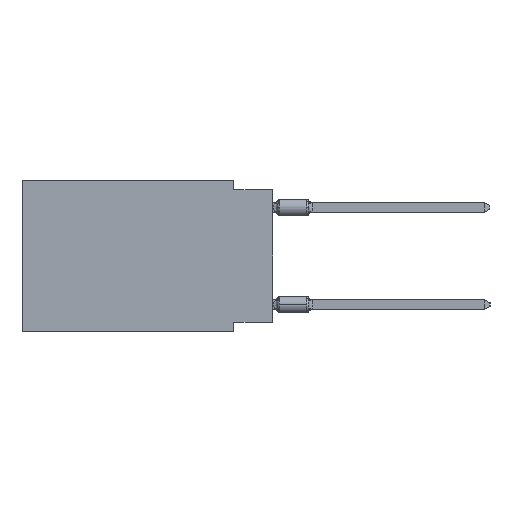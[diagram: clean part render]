
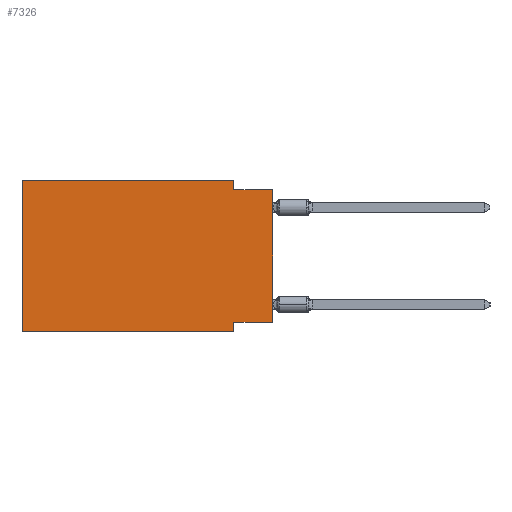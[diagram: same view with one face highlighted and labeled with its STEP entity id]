
A CAD part, left-side view. The second image highlights one B-rep face of the part: STEP entity #7326.
In plain terms, the highlighted planar face has unit normal (-1, 0, 0).
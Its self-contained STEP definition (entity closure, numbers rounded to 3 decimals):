
#221 = FACE_OUTER_BOUND ( 'NONE', #14577, .T. ) ;
#723 = VERTEX_POINT ( 'NONE', #28450 ) ;
#2229 = VECTOR ( 'NONE', #12782, 1000. ) ;
#2378 = ORIENTED_EDGE ( 'NONE', *, *, #22468, .F. ) ;
#6672 = VECTOR ( 'NONE', #10635, 1000. ) ;
#6762 = CARTESIAN_POINT ( 'NONE',  ( 0., 16.383, -9.906 ) ) ;
#6782 = LINE ( 'NONE', #16439, #27927 ) ;
#7326 = ADVANCED_FACE ( 'NONE', ( #221 ), #36456, .F. ) ;
#7365 = CARTESIAN_POINT ( 'NONE',  ( 0., 0., -0.635 ) ) ;
#8652 = ORIENTED_EDGE ( 'NONE', *, *, #21023, .F. ) ;
#9403 = VECTOR ( 'NONE', #28242, 1000. ) ;
#9588 = LINE ( 'NONE', #32516, #9403 ) ;
#9988 = EDGE_CURVE ( 'NONE', #11598, #723, #24041, .T. ) ;
#10635 = DIRECTION ( 'NONE',  ( 0., 0., 1. ) ) ;
#10671 = ORIENTED_EDGE ( 'NONE', *, *, #22669, .T. ) ;
#11536 = AXIS2_PLACEMENT_3D ( 'NONE', #39696, #36029, #13299 ) ;
#11598 = VERTEX_POINT ( 'NONE', #26790 ) ;
#11689 = ORIENTED_EDGE ( 'NONE', *, *, #31273, .T. ) ;
#12542 = CARTESIAN_POINT ( 'NONE',  ( 0., 16.383, -9.906 ) ) ;
#12782 = DIRECTION ( 'NONE',  ( 0., 0., 1. ) ) ;
#13299 = DIRECTION ( 'NONE',  ( 0., 0., -1. ) ) ;
#13474 = ORIENTED_EDGE ( 'NONE', *, *, #22496, .F. ) ;
#14577 = EDGE_LOOP ( 'NONE', ( #11689, #2378, #8652, #30738, #13474, #10671, #21181, #32651 ) ) ;
#14647 = CARTESIAN_POINT ( 'NONE',  ( 0., 0., -9.271 ) ) ;
#15117 = DIRECTION ( 'NONE',  ( 0., -1., 0. ) ) ;
#15350 = VERTEX_POINT ( 'NONE', #32488 ) ;
#16439 = CARTESIAN_POINT ( 'NONE',  ( 0., 0., -0.635 ) ) ;
#16622 = VERTEX_POINT ( 'NONE', #6762 ) ;
#17431 = VERTEX_POINT ( 'NONE', #36256 ) ;
#17753 = DIRECTION ( 'NONE',  ( 0., 0., -1. ) ) ;
#21023 = EDGE_CURVE ( 'NONE', #723, #17431, #34037, .T. ) ;
#21181 = ORIENTED_EDGE ( 'NONE', *, *, #34176, .F. ) ;
#22374 = EDGE_CURVE ( 'NONE', #24174, #34410, #9588, .T. ) ;
#22468 = EDGE_CURVE ( 'NONE', #17431, #40399, #6782, .T. ) ;
#22476 = LINE ( 'NONE', #37910, #37982 ) ;
#22496 = EDGE_CURVE ( 'NONE', #16622, #11598, #33362, .T. ) ;
#22669 = EDGE_CURVE ( 'NONE', #16622, #15350, #28402, .T. ) ;
#24006 = VECTOR ( 'NONE', #33677, 1000. ) ;
#24041 = LINE ( 'NONE', #27251, #24006 ) ;
#24174 = VERTEX_POINT ( 'NONE', #14647 ) ;
#26790 = CARTESIAN_POINT ( 'NONE',  ( 0., 16.383, 0. ) ) ;
#27251 = CARTESIAN_POINT ( 'NONE',  ( 0., 16.383, 0. ) ) ;
#27638 = VECTOR ( 'NONE', #17753, 1000. ) ;
#27927 = VECTOR ( 'NONE', #29510, 1000. ) ;
#28242 = DIRECTION ( 'NONE',  ( 0., 1., 0. ) ) ;
#28257 = DIRECTION ( 'NONE',  ( 0., 0., -1. ) ) ;
#28402 = LINE ( 'NONE', #12542, #36117 ) ;
#28431 = LINE ( 'NONE', #32089, #2229 ) ;
#28450 = CARTESIAN_POINT ( 'NONE',  ( 0., 2.54, 0. ) ) ;
#29311 = CARTESIAN_POINT ( 'NONE',  ( 0., 16.383, 0. ) ) ;
#29510 = DIRECTION ( 'NONE',  ( 0., -1., 0. ) ) ;
#30738 = ORIENTED_EDGE ( 'NONE', *, *, #9988, .F. ) ;
#31273 = EDGE_CURVE ( 'NONE', #24174, #40399, #28431, .T. ) ;
#32089 = CARTESIAN_POINT ( 'NONE',  ( 0., 0., 0. ) ) ;
#32488 = CARTESIAN_POINT ( 'NONE',  ( 0., 2.54, -9.906 ) ) ;
#32516 = CARTESIAN_POINT ( 'NONE',  ( 0., 0., -9.271 ) ) ;
#32651 = ORIENTED_EDGE ( 'NONE', *, *, #22374, .F. ) ;
#33362 = LINE ( 'NONE', #29311, #6672 ) ;
#33621 = CARTESIAN_POINT ( 'NONE',  ( 0., 2.54, 0. ) ) ;
#33677 = DIRECTION ( 'NONE',  ( 0., -1., 0. ) ) ;
#34037 = LINE ( 'NONE', #33621, #27638 ) ;
#34176 = EDGE_CURVE ( 'NONE', #34410, #15350, #22476, .T. ) ;
#34410 = VERTEX_POINT ( 'NONE', #40664 ) ;
#36029 = DIRECTION ( 'NONE',  ( 1., 0., 0. ) ) ;
#36117 = VECTOR ( 'NONE', #15117, 1000. ) ;
#36256 = CARTESIAN_POINT ( 'NONE',  ( 0., 2.54, -0.635 ) ) ;
#36456 = PLANE ( 'NONE',  #11536 ) ;
#37910 = CARTESIAN_POINT ( 'NONE',  ( 0., 2.54, -9.906 ) ) ;
#37982 = VECTOR ( 'NONE', #28257, 1000. ) ;
#39696 = CARTESIAN_POINT ( 'NONE',  ( 0., 16.383, 0. ) ) ;
#40399 = VERTEX_POINT ( 'NONE', #7365 ) ;
#40664 = CARTESIAN_POINT ( 'NONE',  ( 0., 2.54, -9.271 ) ) ;
